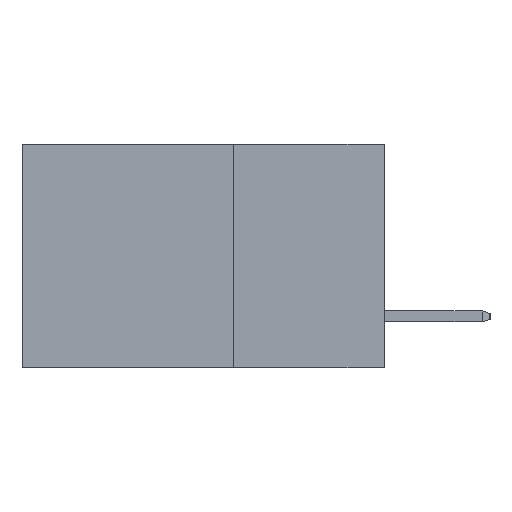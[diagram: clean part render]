
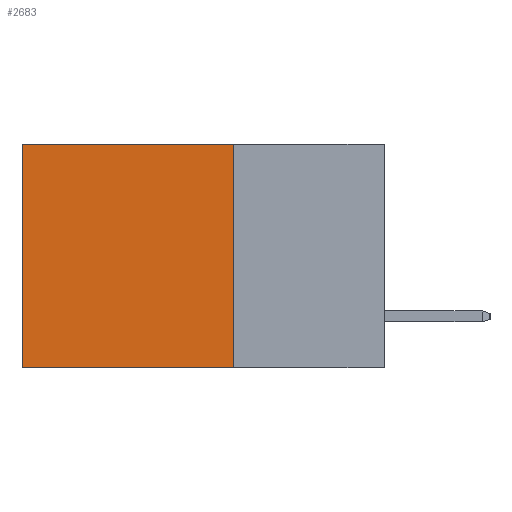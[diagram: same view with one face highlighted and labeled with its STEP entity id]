
A CAD part, left-side view. The second image highlights one B-rep face of the part: STEP entity #2683.
In plain terms, the highlighted planar face has unit normal (-1, 0, 0).
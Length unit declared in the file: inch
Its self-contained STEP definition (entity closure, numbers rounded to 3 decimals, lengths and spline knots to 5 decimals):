
#255 = CARTESIAN_POINT ( 'NONE',  ( 0.2615, 0.25, 0. ) ) ;
#309 = LINE ( 'NONE', #255, #6048 ) ;
#466 = DIRECTION ( 'NONE',  ( 0., 0., -1. ) ) ;
#486 = DIRECTION ( 'NONE',  ( 1., 0., 0. ) ) ;
#544 = ORIENTED_EDGE ( 'NONE', *, *, #1208, .F. ) ;
#665 = CARTESIAN_POINT ( 'NONE',  ( 0.2615, 0.25, -0.37 ) ) ;
#900 = EDGE_CURVE ( 'NONE', #1780, #3841, #2341, .T. ) ;
#901 = PLANE ( 'NONE',  #6438 ) ;
#1208 = EDGE_CURVE ( 'NONE', #3841, #2209, #1751, .T. ) ;
#1678 = DIRECTION ( 'NONE',  ( 0., 1., 0. ) ) ;
#1751 = LINE ( 'NONE', #3317, #9247 ) ;
#1780 = VERTEX_POINT ( 'NONE', #6806 ) ;
#2209 = VERTEX_POINT ( 'NONE', #9364 ) ;
#2341 = LINE ( 'NONE', #6601, #6172 ) ;
#2462 = EDGE_CURVE ( 'NONE', #3426, #2209, #6929, .T. ) ;
#2473 = ORIENTED_EDGE ( 'NONE', *, *, #900, .F. ) ;
#2683 = ADVANCED_FACE ( 'NONE', ( #6139 ), #901, .F. ) ;
#3317 = CARTESIAN_POINT ( 'NONE',  ( 0.2615, 0.25, -0.37 ) ) ;
#3426 = VERTEX_POINT ( 'NONE', #6719 ) ;
#3841 = VERTEX_POINT ( 'NONE', #8053 ) ;
#3932 = DIRECTION ( 'NONE',  ( 0., 0., -1. ) ) ;
#3982 = CARTESIAN_POINT ( 'NONE',  ( 0.2615, 0.6, -0.37 ) ) ;
#4612 = ORIENTED_EDGE ( 'NONE', *, *, #6521, .T. ) ;
#4851 = DIRECTION ( 'NONE',  ( 0., 0., -1. ) ) ;
#5868 = EDGE_LOOP ( 'NONE', ( #6280, #544, #2473, #4612 ) ) ;
#6048 = VECTOR ( 'NONE', #1678, 39.37008 ) ;
#6139 = FACE_OUTER_BOUND ( 'NONE', #5868, .T. ) ;
#6172 = VECTOR ( 'NONE', #4851, 39.37008 ) ;
#6280 = ORIENTED_EDGE ( 'NONE', *, *, #2462, .T. ) ;
#6438 = AXIS2_PLACEMENT_3D ( 'NONE', #665, #486, #466 ) ;
#6521 = EDGE_CURVE ( 'NONE', #1780, #3426, #309, .T. ) ;
#6601 = CARTESIAN_POINT ( 'NONE',  ( 0.2615, 0.25, -0.37 ) ) ;
#6719 = CARTESIAN_POINT ( 'NONE',  ( 0.2615, 0.6, 0. ) ) ;
#6806 = CARTESIAN_POINT ( 'NONE',  ( 0.2615, 0.25, 0. ) ) ;
#6929 = LINE ( 'NONE', #3982, #8707 ) ;
#8053 = CARTESIAN_POINT ( 'NONE',  ( 0.2615, 0.25, -0.37 ) ) ;
#8303 = DIRECTION ( 'NONE',  ( 0., 1., 0. ) ) ;
#8707 = VECTOR ( 'NONE', #3932, 39.37008 ) ;
#9247 = VECTOR ( 'NONE', #8303, 39.37008 ) ;
#9364 = CARTESIAN_POINT ( 'NONE',  ( 0.2615, 0.6, -0.37 ) ) ;
